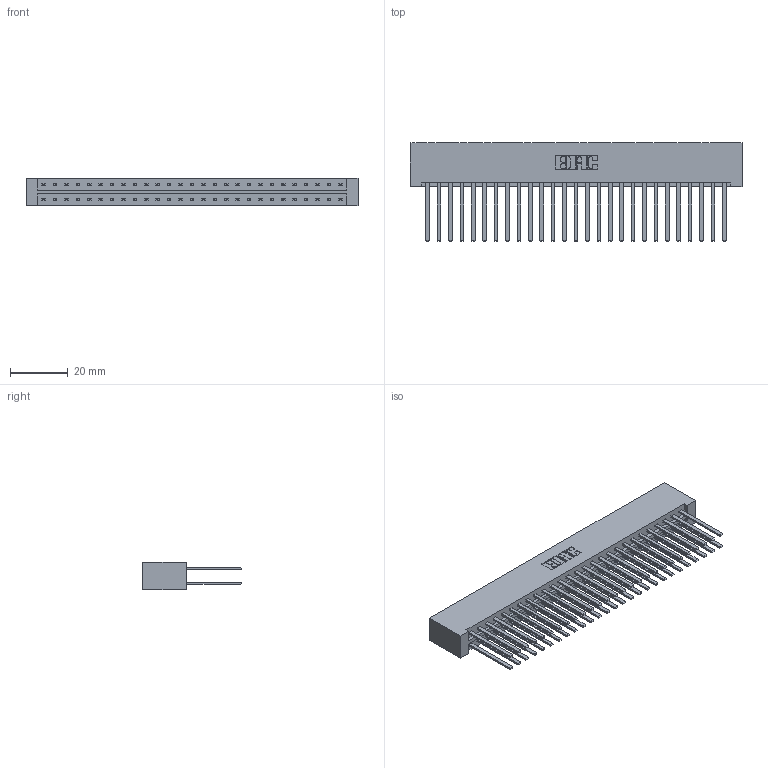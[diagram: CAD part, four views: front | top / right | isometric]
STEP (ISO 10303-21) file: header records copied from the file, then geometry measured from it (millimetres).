
FILE_DESCRIPTION (( 'STEP AP203' ), '1' );
FILE_NAME ('833-054-544-201.STEP', '2020-06-04T21:13:30', ( '' ), ( '' ), 'SwSTEP 2.0', 'SolidWorks 2020', '' );
FILE_SCHEMA (( 'CONFIG_CONTROL_DESIGN' ));
Length unit declared in the file: inch
Products named in the file (3): 833 Part_Lugless; 345-292-001_345-293-144; 833-054-544-201
Assembly tree (55 placements, depth 2):
  833-054-544-201
    833 Part_Lugless
    345-292-001_345-293-144  x54
Bounding box: 115.24 x 34.3 x 9.4 mm (x, y, z)
Volume: 13014.3 mm3; surface area: 17686.5 mm2
Topology: 55 solids, 55 shells, 2590 faces, 7685 edges, 5050 vertices
Faces by surface type: plane 1794, cylinder 796
Entity records: 18849 total; most frequent: CARTESIAN_POINT 3138, ORIENTED_EDGE 3074, DIRECTION 2697, EDGE_CURVE 1537, LINE 1421, VECTOR 1421, VERTEX_POINT 1022, AXIS2_PLACEMENT_3D 638
